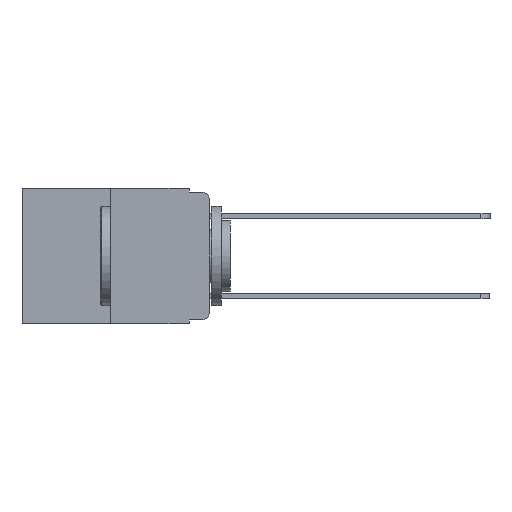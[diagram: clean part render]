
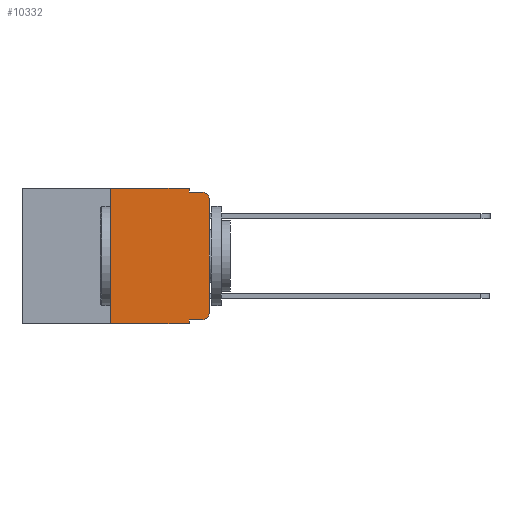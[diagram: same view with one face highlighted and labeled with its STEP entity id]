
A CAD part, left-side view. The second image highlights one B-rep face of the part: STEP entity #10332.
In plain terms, the highlighted planar face has unit normal (-1, 0, 0).
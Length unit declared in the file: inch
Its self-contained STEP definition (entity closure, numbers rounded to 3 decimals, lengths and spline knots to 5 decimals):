
#169 = AXIS2_PLACEMENT_3D ( 'NONE', #3685, #15308, #6655 ) ;
#366 = VERTEX_POINT ( 'NONE', #11508 ) ;
#997 = VERTEX_POINT ( 'NONE', #4137 ) ;
#1169 = VERTEX_POINT ( 'NONE', #15756 ) ;
#1286 = DIRECTION ( 'NONE',  ( 0., 0., 1. ) ) ;
#1476 = ORIENTED_EDGE ( 'NONE', *, *, #12321, .T. ) ;
#1779 = EDGE_CURVE ( 'NONE', #17593, #1169, #18617, .T. ) ;
#2189 = EDGE_LOOP ( 'NONE', ( #5701, #17010, #18770, #13213, #16391, #6244, #12811, #11990, #18038, #1476 ) ) ;
#2243 = DIRECTION ( 'NONE',  ( -1., 0., 0. ) ) ;
#2717 = DIRECTION ( 'NONE',  ( 0., 0., -1. ) ) ;
#3409 = EDGE_CURVE ( 'NONE', #17593, #16272, #5953, .T. ) ;
#3685 = CARTESIAN_POINT ( 'NONE',  ( 0., 0.473, 0. ) ) ;
#3908 = CARTESIAN_POINT ( 'NONE',  ( 0., 0., 0. ) ) ;
#4076 = CARTESIAN_POINT ( 'NONE',  ( 0., 0.051, -0.333 ) ) ;
#4137 = CARTESIAN_POINT ( 'NONE',  ( 0., 0., -0.313 ) ) ;
#4251 = EDGE_CURVE ( 'NONE', #997, #8079, #18298, .T. ) ;
#4491 = EDGE_CURVE ( 'NONE', #12319, #10051, #18514, .T. ) ;
#4804 = CARTESIAN_POINT ( 'NONE',  ( 0., 0.051, -0.01 ) ) ;
#5016 = EDGE_CURVE ( 'NONE', #12343, #7472, #5649, .T. ) ;
#5649 = LINE ( 'NONE', #5685, #16731 ) ;
#5685 = CARTESIAN_POINT ( 'NONE',  ( 0., 0.051, -0.01 ) ) ;
#5701 = ORIENTED_EDGE ( 'NONE', *, *, #4251, .T. ) ;
#5765 = VECTOR ( 'NONE', #10908, 39.37008 ) ;
#5905 = DIRECTION ( 'NONE',  ( 0., -1., 0. ) ) ;
#5953 = LINE ( 'NONE', #9435, #13200 ) ;
#6225 = DIRECTION ( 'NONE',  ( -1., 0., 0. ) ) ;
#6244 = ORIENTED_EDGE ( 'NONE', *, *, #12794, .F. ) ;
#6655 = DIRECTION ( 'NONE',  ( 0., 0., -1. ) ) ;
#6714 = CARTESIAN_POINT ( 'NONE',  ( 0., 0., -0.03 ) ) ;
#7472 = VERTEX_POINT ( 'NONE', #11109 ) ;
#7503 = VECTOR ( 'NONE', #2717, 39.37008 ) ;
#7605 = VECTOR ( 'NONE', #16205, 39.37008 ) ;
#7953 = DIRECTION ( 'NONE',  ( 0., 0., -1. ) ) ;
#8059 = CARTESIAN_POINT ( 'NONE',  ( 0., 0.473, -0.343 ) ) ;
#8079 = VERTEX_POINT ( 'NONE', #6714 ) ;
#8626 = VECTOR ( 'NONE', #1286, 39.37008 ) ;
#8985 = CIRCLE ( 'NONE', #16483, 0.02 ) ;
#9435 = CARTESIAN_POINT ( 'NONE',  ( 0., 0.051, 0. ) ) ;
#9704 = EDGE_CURVE ( 'NONE', #366, #16272, #17724, .T. ) ;
#9970 = CARTESIAN_POINT ( 'NONE',  ( 0., 0.051, -0.333 ) ) ;
#10025 = CARTESIAN_POINT ( 'NONE',  ( 0., 0.051, 0. ) ) ;
#10051 = VERTEX_POINT ( 'NONE', #17514 ) ;
#10078 = DIRECTION ( 'NONE',  ( 0., -1., 0. ) ) ;
#10286 = CARTESIAN_POINT ( 'NONE',  ( 0., 0.473, 0. ) ) ;
#10332 = ADVANCED_FACE ( 'NONE', ( #14596 ), #13859, .F. ) ;
#10682 = VECTOR ( 'NONE', #12620, 39.37008 ) ;
#10908 = DIRECTION ( 'NONE',  ( 0., -1., 0. ) ) ;
#11008 = CARTESIAN_POINT ( 'NONE',  ( 0., 0.02, -0.03 ) ) ;
#11109 = CARTESIAN_POINT ( 'NONE',  ( 0., 0.02, -0.01 ) ) ;
#11349 = LINE ( 'NONE', #10025, #7503 ) ;
#11508 = CARTESIAN_POINT ( 'NONE',  ( 0., 0.25, -0.343 ) ) ;
#11828 = EDGE_CURVE ( 'NONE', #10051, #12343, #11349, .T. ) ;
#11990 = ORIENTED_EDGE ( 'NONE', *, *, #3409, .F. ) ;
#12027 = CIRCLE ( 'NONE', #14650, 0.02 ) ;
#12319 = VERTEX_POINT ( 'NONE', #16278 ) ;
#12321 = EDGE_CURVE ( 'NONE', #1169, #997, #12027, .T. ) ;
#12343 = VERTEX_POINT ( 'NONE', #4804 ) ;
#12466 = LINE ( 'NONE', #18648, #8626 ) ;
#12470 = DIRECTION ( 'NONE',  ( 0., 0., -1. ) ) ;
#12620 = DIRECTION ( 'NONE',  ( 0., 0., 1. ) ) ;
#12794 = EDGE_CURVE ( 'NONE', #366, #12319, #12466, .T. ) ;
#12811 = ORIENTED_EDGE ( 'NONE', *, *, #9704, .T. ) ;
#13200 = VECTOR ( 'NONE', #7953, 39.37008 ) ;
#13213 = ORIENTED_EDGE ( 'NONE', *, *, #11828, .F. ) ;
#13859 = PLANE ( 'NONE',  #169 ) ;
#14288 = VECTOR ( 'NONE', #5905, 39.37008 ) ;
#14596 = FACE_OUTER_BOUND ( 'NONE', #2189, .T. ) ;
#14650 = AXIS2_PLACEMENT_3D ( 'NONE', #14876, #6225, #16335 ) ;
#14876 = CARTESIAN_POINT ( 'NONE',  ( 0., 0.02, -0.313 ) ) ;
#15308 = DIRECTION ( 'NONE',  ( 1., 0., 0. ) ) ;
#15670 = EDGE_CURVE ( 'NONE', #8079, #7472, #8985, .T. ) ;
#15756 = CARTESIAN_POINT ( 'NONE',  ( 0., 0.02, -0.333 ) ) ;
#16205 = DIRECTION ( 'NONE',  ( 0., -1., 0. ) ) ;
#16272 = VERTEX_POINT ( 'NONE', #18007 ) ;
#16278 = CARTESIAN_POINT ( 'NONE',  ( 0., 0.25, 0. ) ) ;
#16335 = DIRECTION ( 'NONE',  ( 0., 0., -1. ) ) ;
#16391 = ORIENTED_EDGE ( 'NONE', *, *, #4491, .F. ) ;
#16483 = AXIS2_PLACEMENT_3D ( 'NONE', #11008, #2243, #12470 ) ;
#16731 = VECTOR ( 'NONE', #10078, 39.37008 ) ;
#17010 = ORIENTED_EDGE ( 'NONE', *, *, #15670, .T. ) ;
#17514 = CARTESIAN_POINT ( 'NONE',  ( 0., 0.051, 0. ) ) ;
#17593 = VERTEX_POINT ( 'NONE', #4076 ) ;
#17724 = LINE ( 'NONE', #8059, #5765 ) ;
#18007 = CARTESIAN_POINT ( 'NONE',  ( 0., 0.051, -0.343 ) ) ;
#18038 = ORIENTED_EDGE ( 'NONE', *, *, #1779, .T. ) ;
#18298 = LINE ( 'NONE', #3908, #10682 ) ;
#18514 = LINE ( 'NONE', #10286, #14288 ) ;
#18617 = LINE ( 'NONE', #9970, #7605 ) ;
#18648 = CARTESIAN_POINT ( 'NONE',  ( 0., 0.25, 0. ) ) ;
#18770 = ORIENTED_EDGE ( 'NONE', *, *, #5016, .F. ) ;
